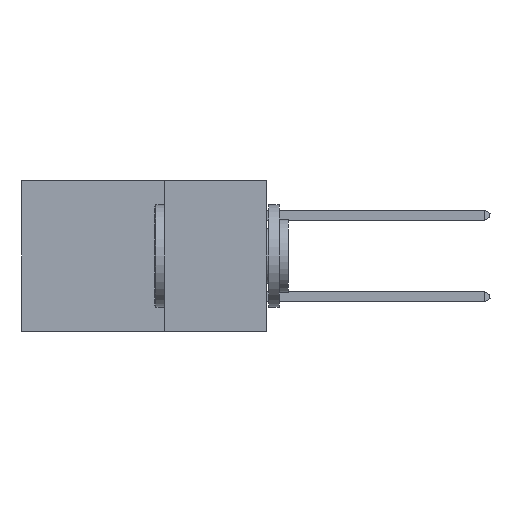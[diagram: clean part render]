
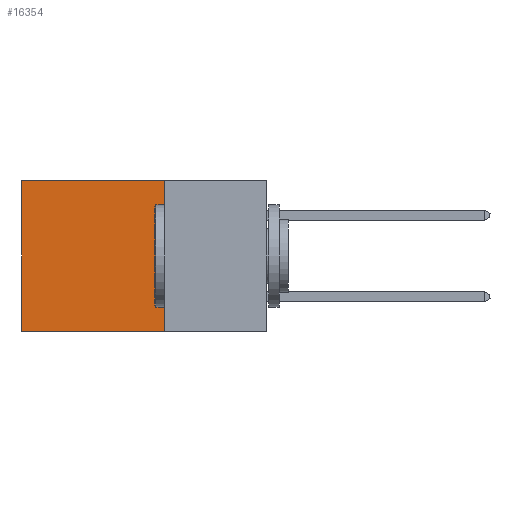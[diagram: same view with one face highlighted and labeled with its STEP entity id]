
A CAD part, left-side view. The second image highlights one B-rep face of the part: STEP entity #16354.
In plain terms, the highlighted planar face has unit normal (-1, 0, 0).
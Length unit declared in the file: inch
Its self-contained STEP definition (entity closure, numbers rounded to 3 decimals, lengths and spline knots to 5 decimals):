
#371 = VERTEX_POINT ( 'NONE', #2253 ) ;
#827 = DIRECTION ( 'NONE',  ( 0., 1., 0. ) ) ;
#862 = CARTESIAN_POINT ( 'NONE',  ( 0.2875, 0.25, -0.37 ) ) ;
#1183 = PLANE ( 'NONE',  #1983 ) ;
#1983 = AXIS2_PLACEMENT_3D ( 'NONE', #10990, #2605, #12400 ) ;
#2253 = CARTESIAN_POINT ( 'NONE',  ( 0.2875, 0.6, 0. ) ) ;
#2562 = CARTESIAN_POINT ( 'NONE',  ( 0.2875, 0.25, 0. ) ) ;
#2605 = DIRECTION ( 'NONE',  ( 1., 0., 0. ) ) ;
#2880 = CARTESIAN_POINT ( 'NONE',  ( 0.2875, 0.25, 0. ) ) ;
#3684 = CARTESIAN_POINT ( 'NONE',  ( 0.2875, 0.25, 0. ) ) ;
#4279 = EDGE_CURVE ( 'NONE', #11901, #12259, #7806, .T. ) ;
#4289 = LINE ( 'NONE', #3684, #7972 ) ;
#5272 = CARTESIAN_POINT ( 'NONE',  ( 0.2875, 0.6, -0.37 ) ) ;
#7232 = VECTOR ( 'NONE', #13911, 39.37008 ) ;
#7364 = VECTOR ( 'NONE', #827, 39.37008 ) ;
#7677 = ORIENTED_EDGE ( 'NONE', *, *, #10031, .T. ) ;
#7806 = LINE ( 'NONE', #862, #7364 ) ;
#7972 = VECTOR ( 'NONE', #16181, 39.37008 ) ;
#8131 = EDGE_LOOP ( 'NONE', ( #7677, #11289, #9363, #10130 ) ) ;
#8909 = VERTEX_POINT ( 'NONE', #2880 ) ;
#9363 = ORIENTED_EDGE ( 'NONE', *, *, #15757, .F. ) ;
#9698 = CARTESIAN_POINT ( 'NONE',  ( 0.2875, 0.6, 0. ) ) ;
#10006 = VECTOR ( 'NONE', #11009, 39.37008 ) ;
#10031 = EDGE_CURVE ( 'NONE', #371, #12259, #17014, .T. ) ;
#10130 = ORIENTED_EDGE ( 'NONE', *, *, #17404, .T. ) ;
#10990 = CARTESIAN_POINT ( 'NONE',  ( 0.2875, 0.25, 0. ) ) ;
#11009 = DIRECTION ( 'NONE',  ( 0., 0., -1. ) ) ;
#11289 = ORIENTED_EDGE ( 'NONE', *, *, #4279, .F. ) ;
#11901 = VERTEX_POINT ( 'NONE', #16333 ) ;
#12259 = VERTEX_POINT ( 'NONE', #5272 ) ;
#12400 = DIRECTION ( 'NONE',  ( 0., 0., -1. ) ) ;
#13911 = DIRECTION ( 'NONE',  ( 0., 0., -1. ) ) ;
#14159 = LINE ( 'NONE', #2562, #10006 ) ;
#15757 = EDGE_CURVE ( 'NONE', #8909, #11901, #14159, .T. ) ;
#16181 = DIRECTION ( 'NONE',  ( 0., 1., 0. ) ) ;
#16333 = CARTESIAN_POINT ( 'NONE',  ( 0.2875, 0.25, -0.37 ) ) ;
#16354 = ADVANCED_FACE ( 'NONE', ( #17556 ), #1183, .F. ) ;
#17014 = LINE ( 'NONE', #9698, #7232 ) ;
#17404 = EDGE_CURVE ( 'NONE', #8909, #371, #4289, .T. ) ;
#17556 = FACE_OUTER_BOUND ( 'NONE', #8131, .T. ) ;
